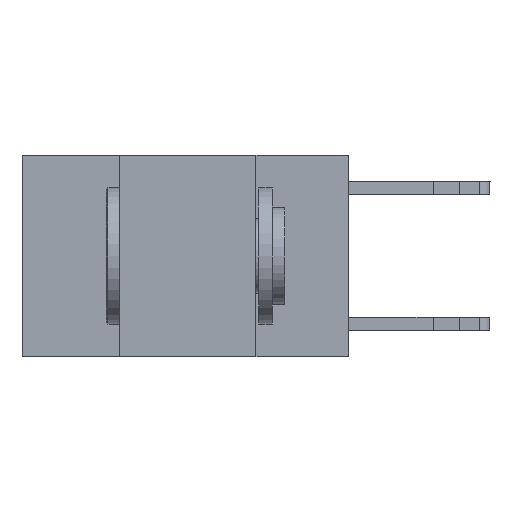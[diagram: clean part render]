
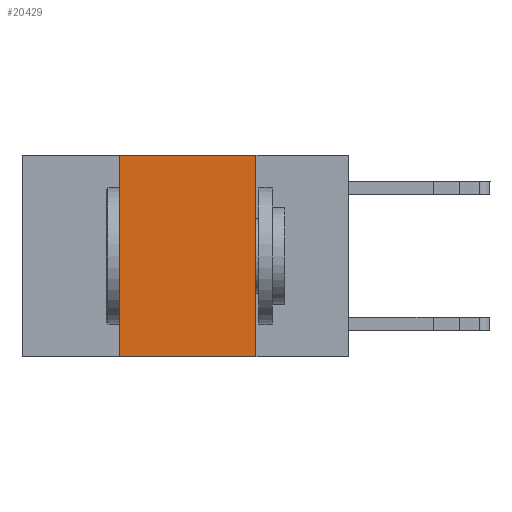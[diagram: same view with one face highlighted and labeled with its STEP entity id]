
A CAD part, left-side view. The second image highlights one B-rep face of the part: STEP entity #20429.
In plain terms, the highlighted planar face has unit normal (-1, 0, 0).
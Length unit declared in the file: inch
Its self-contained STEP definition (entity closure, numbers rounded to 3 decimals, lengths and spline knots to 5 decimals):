
#1346 = DIRECTION ( 'NONE',  ( 0., 0., -1. ) ) ;
#1953 = FACE_OUTER_BOUND ( 'NONE', #24258, .T. ) ;
#2521 = ORIENTED_EDGE ( 'NONE', *, *, #8441, .F. ) ;
#3420 = CARTESIAN_POINT ( 'NONE',  ( 0., 0.17, 0. ) ) ;
#5285 = CARTESIAN_POINT ( 'NONE',  ( 0., 0.42, 0. ) ) ;
#5460 = CARTESIAN_POINT ( 'NONE',  ( 0., 0.6, 0. ) ) ;
#5729 = DIRECTION ( 'NONE',  ( 0., -1., 0. ) ) ;
#6212 = VECTOR ( 'NONE', #5729, 39.37008 ) ;
#7793 = ORIENTED_EDGE ( 'NONE', *, *, #13377, .F. ) ;
#8018 = DIRECTION ( 'NONE',  ( 0., 0., 1. ) ) ;
#8229 = CARTESIAN_POINT ( 'NONE',  ( 0., 0.6, 0. ) ) ;
#8441 = EDGE_CURVE ( 'NONE', #24625, #11919, #18064, .T. ) ;
#9566 = PLANE ( 'NONE',  #15847 ) ;
#10861 = VECTOR ( 'NONE', #1346, 39.37008 ) ;
#11657 = LINE ( 'NONE', #3420, #10861 ) ;
#11919 = VERTEX_POINT ( 'NONE', #5285 ) ;
#13377 = EDGE_CURVE ( 'NONE', #17217, #21813, #11657, .T. ) ;
#13453 = CARTESIAN_POINT ( 'NONE',  ( 0., 0.6, -0.37 ) ) ;
#13636 = LINE ( 'NONE', #8229, #15525 ) ;
#14093 = CARTESIAN_POINT ( 'NONE',  ( 0., 0.17, -0.37 ) ) ;
#14890 = VECTOR ( 'NONE', #8018, 39.37008 ) ;
#15296 = EDGE_CURVE ( 'NONE', #24625, #21813, #17310, .T. ) ;
#15525 = VECTOR ( 'NONE', #19932, 39.37008 ) ;
#15847 = AXIS2_PLACEMENT_3D ( 'NONE', #5460, #19223, #17671 ) ;
#17217 = VERTEX_POINT ( 'NONE', #19626 ) ;
#17310 = LINE ( 'NONE', #13453, #6212 ) ;
#17671 = DIRECTION ( 'NONE',  ( 0., 0., -1. ) ) ;
#17680 = CARTESIAN_POINT ( 'NONE',  ( 0., 0.42, 0. ) ) ;
#18064 = LINE ( 'NONE', #17680, #14890 ) ;
#19223 = DIRECTION ( 'NONE',  ( 1., 0., 0. ) ) ;
#19626 = CARTESIAN_POINT ( 'NONE',  ( 0., 0.17, 0. ) ) ;
#19932 = DIRECTION ( 'NONE',  ( 0., -1., 0. ) ) ;
#20165 = ORIENTED_EDGE ( 'NONE', *, *, #15296, .T. ) ;
#20229 = ORIENTED_EDGE ( 'NONE', *, *, #24623, .F. ) ;
#20429 = ADVANCED_FACE ( 'NONE', ( #1953 ), #9566, .F. ) ;
#21813 = VERTEX_POINT ( 'NONE', #14093 ) ;
#21893 = CARTESIAN_POINT ( 'NONE',  ( 0., 0.42, -0.37 ) ) ;
#24258 = EDGE_LOOP ( 'NONE', ( #7793, #20229, #2521, #20165 ) ) ;
#24623 = EDGE_CURVE ( 'NONE', #11919, #17217, #13636, .T. ) ;
#24625 = VERTEX_POINT ( 'NONE', #21893 ) ;
